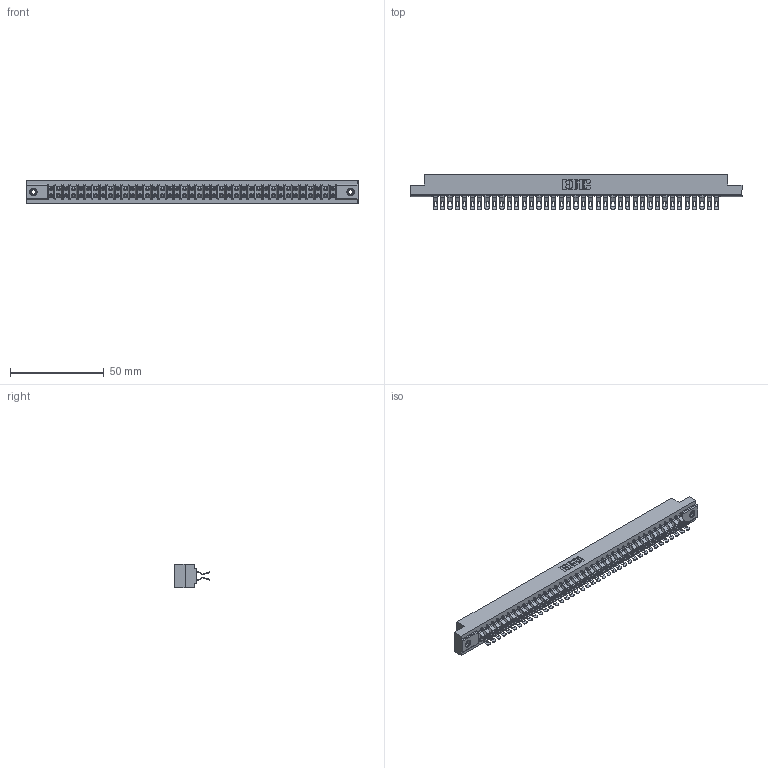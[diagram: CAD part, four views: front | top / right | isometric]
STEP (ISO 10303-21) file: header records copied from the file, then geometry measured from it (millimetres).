
FILE_DESCRIPTION (( 'STEP AP203' ), '1' );
FILE_NAME ('357-078-555-208.STEP', '2019-09-19T14:44:49', ( '' ), ( '' ), 'SwSTEP 2.0', 'SolidWorks 2016', '' );
FILE_SCHEMA (( 'CONFIG_CONTROL_DESIGN' ));
Length unit declared in the file: inch
Products named in the file (4): 307 Part_.156 Dia Mounting Holes; 357-078-555-208; 307-290-001_555; 345-250-001_345-250-003-102
Assembly tree (81 placements, depth 2):
  357-078-555-208
    307 Part_.156 Dia Mounting Holes
    307-290-001_555  x78
    345-250-001_345-250-003-102  x2
Bounding box: 177.55 x 18.75 x 12.7 mm (x, y, z)
Volume: 19084.5 mm3; surface area: 24600.9 mm2
Topology: 81 solids, 81 shells, 4976 faces, 14577 edges, 9498 vertices
Faces by surface type: plane 2754, cylinder 2126, sphere 80, cone 12, torus 4
Entity records: 36774 total; most frequent: CARTESIAN_POINT 6006, ORIENTED_EDGE 5948, DIRECTION 5900, EDGE_CURVE 2974, LINE 2268, VECTOR 2268, VERTEX_POINT 1922, AXIS2_PLACEMENT_3D 1816
